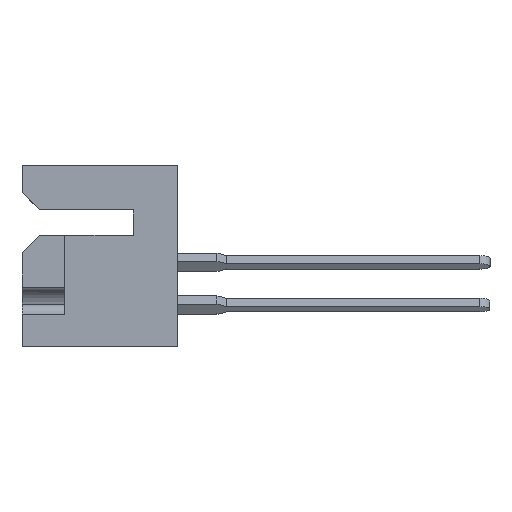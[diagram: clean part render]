
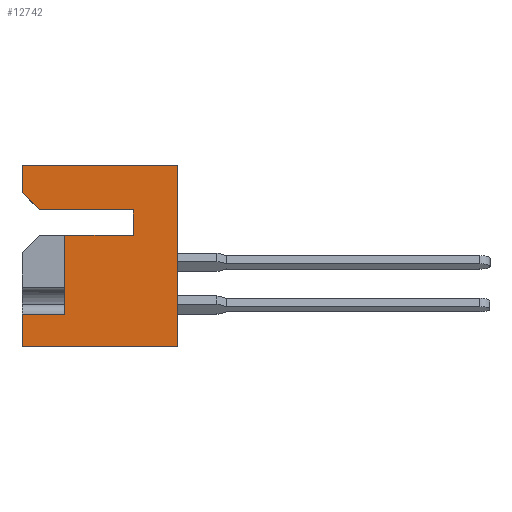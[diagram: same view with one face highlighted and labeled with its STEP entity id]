
A CAD part, left-side view. The second image highlights one B-rep face of the part: STEP entity #12742.
In plain terms, the highlighted planar face has unit normal (-1, 0, 0).
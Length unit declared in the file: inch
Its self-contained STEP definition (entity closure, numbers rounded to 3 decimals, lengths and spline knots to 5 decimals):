
#355 = ORIENTED_EDGE ( 'NONE', *, *, #8004, .F. ) ;
#438 = VECTOR ( 'NONE', #854, 39.37008 ) ;
#583 = CARTESIAN_POINT ( 'NONE',  ( 0., 0.453, 0. ) ) ;
#854 = DIRECTION ( 'NONE',  ( 0., 0., 1. ) ) ;
#1156 = ORIENTED_EDGE ( 'NONE', *, *, #10606, .T. ) ;
#1445 = EDGE_CURVE ( 'NONE', #2015, #3260, #7783, .T. ) ;
#1559 = EDGE_CURVE ( 'NONE', #8086, #2264, #4021, .T. ) ;
#1796 = CARTESIAN_POINT ( 'NONE',  ( 0., 0.128, -0.131 ) ) ;
#2015 = VERTEX_POINT ( 'NONE', #5601 ) ;
#2078 = CARTESIAN_POINT ( 'NONE',  ( 0., 0., 0. ) ) ;
#2264 = VERTEX_POINT ( 'NONE', #10043 ) ;
#2359 = VECTOR ( 'NONE', #7843, 39.37008 ) ;
#2462 = CARTESIAN_POINT ( 'NONE',  ( 0., 0.453, 0. ) ) ;
#2669 = EDGE_CURVE ( 'NONE', #11678, #3260, #10729, .T. ) ;
#2703 = DIRECTION ( 'NONE',  ( 0., 1., 0. ) ) ;
#3260 = VERTEX_POINT ( 'NONE', #6338 ) ;
#3646 = LINE ( 'NONE', #15127, #12779 ) ;
#3744 = VECTOR ( 'NONE', #2703, 39.37008 ) ;
#3822 = EDGE_CURVE ( 'NONE', #8086, #6806, #4931, .T. ) ;
#3918 = ORIENTED_EDGE ( 'NONE', *, *, #5211, .T. ) ;
#4021 = LINE ( 'NONE', #11215, #15893 ) ;
#4254 = DIRECTION ( 'NONE',  ( 0., 0., 1. ) ) ;
#4457 = VERTEX_POINT ( 'NONE', #5586 ) ;
#4580 = DIRECTION ( 'NONE',  ( 0., -0.707, -0.707 ) ) ;
#4931 = LINE ( 'NONE', #5480, #15824 ) ;
#5015 = EDGE_CURVE ( 'NONE', #13734, #9102, #15373, .T. ) ;
#5043 = FACE_OUTER_BOUND ( 'NONE', #15339, .T. ) ;
#5211 = EDGE_CURVE ( 'NONE', #8370, #6328, #12820, .T. ) ;
#5480 = CARTESIAN_POINT ( 'NONE',  ( 0., 0.453, 0. ) ) ;
#5534 = CARTESIAN_POINT ( 'NONE',  ( 0., 0.453, -0.531 ) ) ;
#5586 = CARTESIAN_POINT ( 'NONE',  ( 0., 0.328, -0.437 ) ) ;
#5601 = CARTESIAN_POINT ( 'NONE',  ( 0., 0.453, -0.081 ) ) ;
#5869 = VECTOR ( 'NONE', #9361, 39.37008 ) ;
#6273 = ORIENTED_EDGE ( 'NONE', *, *, #3822, .F. ) ;
#6328 = VERTEX_POINT ( 'NONE', #8244 ) ;
#6338 = CARTESIAN_POINT ( 'NONE',  ( 0., 0.403, -0.131 ) ) ;
#6406 = LINE ( 'NONE', #11737, #11565 ) ;
#6658 = CARTESIAN_POINT ( 'NONE',  ( 0., 0., 0. ) ) ;
#6741 = CARTESIAN_POINT ( 'NONE',  ( 0., 0.453, 0. ) ) ;
#6806 = VERTEX_POINT ( 'NONE', #7748 ) ;
#6829 = DIRECTION ( 'NONE',  ( 0., 0., -1. ) ) ;
#7097 = ORIENTED_EDGE ( 'NONE', *, *, #8427, .F. ) ;
#7620 = CARTESIAN_POINT ( 'NONE',  ( 0., 0.128, -0.131 ) ) ;
#7707 = CARTESIAN_POINT ( 'NONE',  ( 0., 0.328, -0.437 ) ) ;
#7748 = CARTESIAN_POINT ( 'NONE',  ( 0., 0.453, -0.437 ) ) ;
#7783 = LINE ( 'NONE', #14687, #12544 ) ;
#7843 = DIRECTION ( 'NONE',  ( 0., 1., 0. ) ) ;
#7917 = ORIENTED_EDGE ( 'NONE', *, *, #1445, .T. ) ;
#8004 = EDGE_CURVE ( 'NONE', #8370, #11678, #16088, .T. ) ;
#8086 = VERTEX_POINT ( 'NONE', #5534 ) ;
#8244 = CARTESIAN_POINT ( 'NONE',  ( 0., 0.328, -0.205 ) ) ;
#8370 = VERTEX_POINT ( 'NONE', #10189 ) ;
#8427 = EDGE_CURVE ( 'NONE', #4457, #6328, #6406, .T. ) ;
#8826 = CARTESIAN_POINT ( 'NONE',  ( 0., 0.128, -0.131 ) ) ;
#8880 = ORIENTED_EDGE ( 'NONE', *, *, #1559, .T. ) ;
#9102 = VERTEX_POINT ( 'NONE', #6658 ) ;
#9361 = DIRECTION ( 'NONE',  ( 0., -1., 0. ) ) ;
#9381 = VECTOR ( 'NONE', #4254, 39.37008 ) ;
#10043 = CARTESIAN_POINT ( 'NONE',  ( 0., 0., -0.531 ) ) ;
#10143 = DIRECTION ( 'NONE',  ( 0., 0., 1. ) ) ;
#10189 = CARTESIAN_POINT ( 'NONE',  ( 0., 0.128, -0.205 ) ) ;
#10366 = ORIENTED_EDGE ( 'NONE', *, *, #13558, .T. ) ;
#10606 = EDGE_CURVE ( 'NONE', #4457, #6806, #14639, .T. ) ;
#10729 = LINE ( 'NONE', #7620, #2359 ) ;
#11201 = ORIENTED_EDGE ( 'NONE', *, *, #5015, .F. ) ;
#11215 = CARTESIAN_POINT ( 'NONE',  ( 0., 0.453, -0.531 ) ) ;
#11565 = VECTOR ( 'NONE', #14261, 39.37008 ) ;
#11678 = VERTEX_POINT ( 'NONE', #8826 ) ;
#11737 = CARTESIAN_POINT ( 'NONE',  ( 0., 0.328, -0.205 ) ) ;
#11973 = DIRECTION ( 'NONE',  ( 0., 0., 1. ) ) ;
#12226 = VECTOR ( 'NONE', #15971, 39.37008 ) ;
#12346 = CARTESIAN_POINT ( 'NONE',  ( 0., 0.128, -0.205 ) ) ;
#12455 = EDGE_CURVE ( 'NONE', #2015, #13734, #3646, .T. ) ;
#12544 = VECTOR ( 'NONE', #4580, 39.37008 ) ;
#12742 = ADVANCED_FACE ( 'NONE', ( #5043 ), #14420, .F. ) ;
#12779 = VECTOR ( 'NONE', #10143, 39.37008 ) ;
#12820 = LINE ( 'NONE', #12346, #12226 ) ;
#12965 = ORIENTED_EDGE ( 'NONE', *, *, #12455, .F. ) ;
#13454 = AXIS2_PLACEMENT_3D ( 'NONE', #6741, #14363, #6829 ) ;
#13558 = EDGE_CURVE ( 'NONE', #2264, #9102, #13899, .T. ) ;
#13734 = VERTEX_POINT ( 'NONE', #2462 ) ;
#13899 = LINE ( 'NONE', #2078, #438 ) ;
#14261 = DIRECTION ( 'NONE',  ( 0., 0., 1. ) ) ;
#14363 = DIRECTION ( 'NONE',  ( 1., 0., 0. ) ) ;
#14420 = PLANE ( 'NONE',  #13454 ) ;
#14442 = ORIENTED_EDGE ( 'NONE', *, *, #2669, .F. ) ;
#14639 = LINE ( 'NONE', #7707, #3744 ) ;
#14687 = CARTESIAN_POINT ( 'NONE',  ( 0., 0.403, -0.131 ) ) ;
#15127 = CARTESIAN_POINT ( 'NONE',  ( 0., 0.453, 0. ) ) ;
#15339 = EDGE_LOOP ( 'NONE', ( #1156, #6273, #8880, #10366, #11201, #12965, #7917, #14442, #355, #3918, #7097 ) ) ;
#15373 = LINE ( 'NONE', #583, #5869 ) ;
#15824 = VECTOR ( 'NONE', #11973, 39.37008 ) ;
#15893 = VECTOR ( 'NONE', #16285, 39.37008 ) ;
#15971 = DIRECTION ( 'NONE',  ( 0., 1., 0. ) ) ;
#16088 = LINE ( 'NONE', #1796, #9381 ) ;
#16285 = DIRECTION ( 'NONE',  ( 0., -1., 0. ) ) ;
